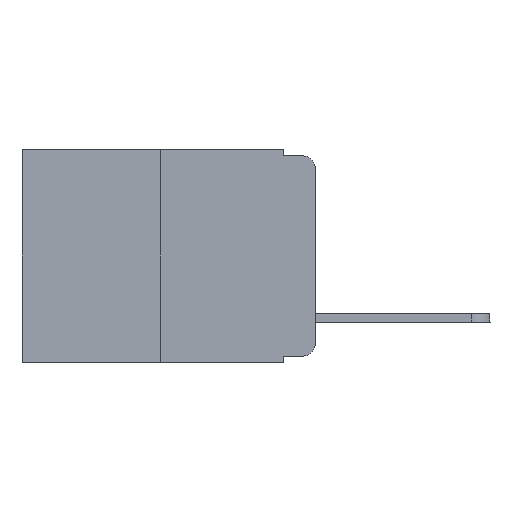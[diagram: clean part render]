
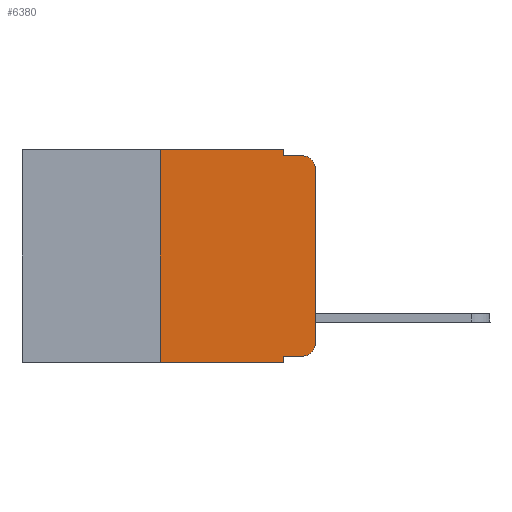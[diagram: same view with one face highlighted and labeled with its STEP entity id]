
A CAD part, left-side view. The second image highlights one B-rep face of the part: STEP entity #6380.
In plain terms, the highlighted planar face has unit normal (-1, 0, 0).
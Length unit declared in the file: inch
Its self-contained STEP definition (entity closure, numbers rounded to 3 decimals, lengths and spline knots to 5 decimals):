
#167 = ORIENTED_EDGE ( 'NONE', *, *, #9188, .F. ) ;
#183 = CARTESIAN_POINT ( 'NONE',  ( 0., 0.02, -0.01 ) ) ;
#354 = EDGE_CURVE ( 'NONE', #10629, #12322, #13641, .T. ) ;
#608 = CARTESIAN_POINT ( 'NONE',  ( 0., 0., -0.313 ) ) ;
#694 = EDGE_CURVE ( 'NONE', #3682, #2411, #5957, .T. ) ;
#753 = VECTOR ( 'NONE', #12293, 39.37008 ) ;
#952 = ORIENTED_EDGE ( 'NONE', *, *, #7409, .T. ) ;
#1218 = DIRECTION ( 'NONE',  ( -1., 0., 0. ) ) ;
#1610 = VECTOR ( 'NONE', #12205, 39.37008 ) ;
#1908 = CIRCLE ( 'NONE', #11351, 0.02 ) ;
#1934 = DIRECTION ( 'NONE',  ( 0., 0., -1. ) ) ;
#2190 = VERTEX_POINT ( 'NONE', #5520 ) ;
#2391 = CARTESIAN_POINT ( 'NONE',  ( 0., 0.051, 0. ) ) ;
#2411 = VERTEX_POINT ( 'NONE', #5478 ) ;
#2419 = LINE ( 'NONE', #14174, #3399 ) ;
#2690 = VECTOR ( 'NONE', #8351, 39.37008 ) ;
#2811 = EDGE_CURVE ( 'NONE', #6484, #12322, #2419, .T. ) ;
#2884 = ORIENTED_EDGE ( 'NONE', *, *, #3527, .F. ) ;
#3342 = EDGE_CURVE ( 'NONE', #8204, #14895, #11772, .T. ) ;
#3399 = VECTOR ( 'NONE', #1934, 39.37008 ) ;
#3527 = EDGE_CURVE ( 'NONE', #9781, #8204, #10453, .T. ) ;
#3542 = DIRECTION ( 'NONE',  ( 0., -1., 0. ) ) ;
#3682 = VERTEX_POINT ( 'NONE', #608 ) ;
#4459 = CARTESIAN_POINT ( 'NONE',  ( 0., 0., 0. ) ) ;
#4520 = DIRECTION ( 'NONE',  ( -1., 0., 0. ) ) ;
#4629 = CARTESIAN_POINT ( 'NONE',  ( 0., 0.051, -0.343 ) ) ;
#4842 = CARTESIAN_POINT ( 'NONE',  ( 0., 0.02, -0.313 ) ) ;
#5478 = CARTESIAN_POINT ( 'NONE',  ( 0., 0., -0.03 ) ) ;
#5520 = CARTESIAN_POINT ( 'NONE',  ( 0., 0.02, -0.333 ) ) ;
#5896 = EDGE_CURVE ( 'NONE', #2190, #3682, #11928, .T. ) ;
#5920 = ORIENTED_EDGE ( 'NONE', *, *, #694, .T. ) ;
#5957 = LINE ( 'NONE', #4459, #2690 ) ;
#6083 = DIRECTION ( 'NONE',  ( 0., -1., 0. ) ) ;
#6380 = ADVANCED_FACE ( 'NONE', ( #11349 ), #12034, .F. ) ;
#6393 = DIRECTION ( 'NONE',  ( 0., -1., 0. ) ) ;
#6484 = VERTEX_POINT ( 'NONE', #12350 ) ;
#6494 = CARTESIAN_POINT ( 'NONE',  ( 0., 0.473, -0.343 ) ) ;
#6524 = VERTEX_POINT ( 'NONE', #183 ) ;
#6536 = AXIS2_PLACEMENT_3D ( 'NONE', #4842, #1218, #11627 ) ;
#6922 = EDGE_CURVE ( 'NONE', #10629, #9781, #10192, .T. ) ;
#7185 = VECTOR ( 'NONE', #6393, 39.37008 ) ;
#7247 = CARTESIAN_POINT ( 'NONE',  ( 0., 0.473, 0. ) ) ;
#7294 = VECTOR ( 'NONE', #11295, 39.37008 ) ;
#7409 = EDGE_CURVE ( 'NONE', #2411, #6524, #1908, .T. ) ;
#7442 = CARTESIAN_POINT ( 'NONE',  ( 0., 0.051, 0. ) ) ;
#8005 = VECTOR ( 'NONE', #6083, 39.37008 ) ;
#8204 = VERTEX_POINT ( 'NONE', #2391 ) ;
#8351 = DIRECTION ( 'NONE',  ( 0., 0., 1. ) ) ;
#8398 = DIRECTION ( 'NONE',  ( 1., 0., 0. ) ) ;
#8399 = CARTESIAN_POINT ( 'NONE',  ( 0., 0.051, -0.333 ) ) ;
#9024 = ORIENTED_EDGE ( 'NONE', *, *, #2811, .F. ) ;
#9188 = EDGE_CURVE ( 'NONE', #14895, #6524, #15460, .T. ) ;
#9438 = ORIENTED_EDGE ( 'NONE', *, *, #354, .T. ) ;
#9510 = ORIENTED_EDGE ( 'NONE', *, *, #3342, .F. ) ;
#9556 = CARTESIAN_POINT ( 'NONE',  ( 0., 0.051, -0.01 ) ) ;
#9781 = VERTEX_POINT ( 'NONE', #14419 ) ;
#9925 = LINE ( 'NONE', #8399, #10860 ) ;
#9933 = EDGE_CURVE ( 'NONE', #6484, #2190, #9925, .T. ) ;
#10192 = LINE ( 'NONE', #13388, #753 ) ;
#10453 = LINE ( 'NONE', #7247, #7185 ) ;
#10629 = VERTEX_POINT ( 'NONE', #13815 ) ;
#10860 = VECTOR ( 'NONE', #3542, 39.37008 ) ;
#11295 = DIRECTION ( 'NONE',  ( 0., -1., 0. ) ) ;
#11349 = FACE_OUTER_BOUND ( 'NONE', #13181, .T. ) ;
#11351 = AXIS2_PLACEMENT_3D ( 'NONE', #11850, #4520, #12977 ) ;
#11627 = DIRECTION ( 'NONE',  ( 0., 0., -1. ) ) ;
#11772 = LINE ( 'NONE', #7442, #1610 ) ;
#11850 = CARTESIAN_POINT ( 'NONE',  ( 0., 0.02, -0.03 ) ) ;
#11928 = CIRCLE ( 'NONE', #6536, 0.02 ) ;
#12034 = PLANE ( 'NONE',  #14729 ) ;
#12036 = ORIENTED_EDGE ( 'NONE', *, *, #6922, .F. ) ;
#12205 = DIRECTION ( 'NONE',  ( 0., 0., -1. ) ) ;
#12293 = DIRECTION ( 'NONE',  ( 0., 0., 1. ) ) ;
#12322 = VERTEX_POINT ( 'NONE', #4629 ) ;
#12350 = CARTESIAN_POINT ( 'NONE',  ( 0., 0.051, -0.333 ) ) ;
#12977 = DIRECTION ( 'NONE',  ( 0., 0., -1. ) ) ;
#13022 = ORIENTED_EDGE ( 'NONE', *, *, #9933, .T. ) ;
#13181 = EDGE_LOOP ( 'NONE', ( #5920, #952, #167, #9510, #2884, #12036, #9438, #9024, #13022, #15847 ) ) ;
#13352 = DIRECTION ( 'NONE',  ( 0., 0., -1. ) ) ;
#13388 = CARTESIAN_POINT ( 'NONE',  ( 0., 0.25, 0. ) ) ;
#13641 = LINE ( 'NONE', #6494, #7294 ) ;
#13815 = CARTESIAN_POINT ( 'NONE',  ( 0., 0.25, -0.343 ) ) ;
#14174 = CARTESIAN_POINT ( 'NONE',  ( 0., 0.051, 0. ) ) ;
#14419 = CARTESIAN_POINT ( 'NONE',  ( 0., 0.25, 0. ) ) ;
#14671 = CARTESIAN_POINT ( 'NONE',  ( 0., 0.051, -0.01 ) ) ;
#14729 = AXIS2_PLACEMENT_3D ( 'NONE', #15713, #8398, #13352 ) ;
#14895 = VERTEX_POINT ( 'NONE', #14671 ) ;
#15460 = LINE ( 'NONE', #9556, #8005 ) ;
#15713 = CARTESIAN_POINT ( 'NONE',  ( 0., 0.473, 0. ) ) ;
#15847 = ORIENTED_EDGE ( 'NONE', *, *, #5896, .T. ) ;
